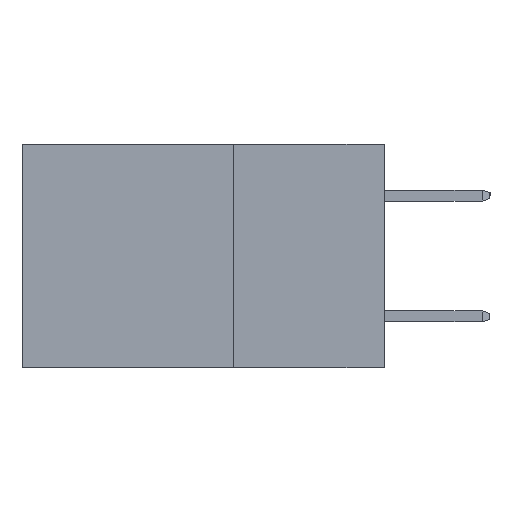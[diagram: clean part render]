
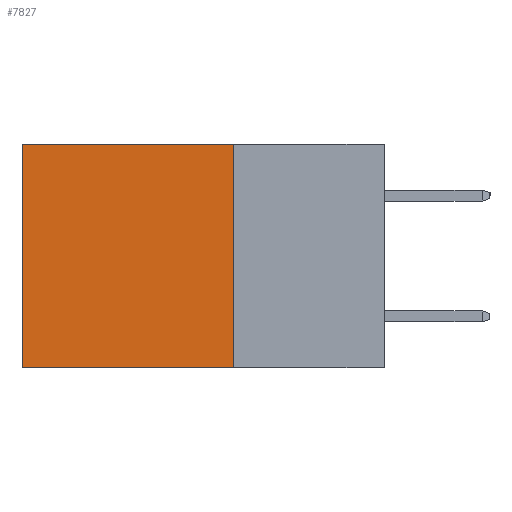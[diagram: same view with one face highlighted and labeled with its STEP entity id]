
A CAD part, left-side view. The second image highlights one B-rep face of the part: STEP entity #7827.
In plain terms, the highlighted planar face has unit normal (-1, 0, 0).
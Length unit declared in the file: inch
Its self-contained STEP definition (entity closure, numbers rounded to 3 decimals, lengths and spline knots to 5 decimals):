
#541 = VECTOR ( 'NONE', #6276, 39.37008 ) ;
#549 = CARTESIAN_POINT ( 'NONE',  ( 0.2615, 0.25, -0.37 ) ) ;
#637 = VERTEX_POINT ( 'NONE', #14362 ) ;
#1221 = VERTEX_POINT ( 'NONE', #3086 ) ;
#1409 = LINE ( 'NONE', #11494, #1584 ) ;
#1584 = VECTOR ( 'NONE', #2761, 39.37008 ) ;
#1722 = AXIS2_PLACEMENT_3D ( 'NONE', #14003, #3047, #11339 ) ;
#1917 = CARTESIAN_POINT ( 'NONE',  ( 0.2615, 0.6, 0. ) ) ;
#2754 = ORIENTED_EDGE ( 'NONE', *, *, #12597, .F. ) ;
#2761 = DIRECTION ( 'NONE',  ( 0., 0., -1. ) ) ;
#3027 = EDGE_LOOP ( 'NONE', ( #10962, #6951, #2754, #10366 ) ) ;
#3047 = DIRECTION ( 'NONE',  ( 1., 0., 0. ) ) ;
#3086 = CARTESIAN_POINT ( 'NONE',  ( 0.2615, 0.25, 0. ) ) ;
#3855 = VECTOR ( 'NONE', #7475, 39.37008 ) ;
#4881 = FACE_OUTER_BOUND ( 'NONE', #3027, .T. ) ;
#5173 = EDGE_CURVE ( 'NONE', #9083, #7657, #5642, .T. ) ;
#5642 = LINE ( 'NONE', #9201, #6374 ) ;
#6276 = DIRECTION ( 'NONE',  ( 0., 1., 0. ) ) ;
#6352 = LINE ( 'NONE', #549, #541 ) ;
#6374 = VECTOR ( 'NONE', #9130, 39.37008 ) ;
#6568 = EDGE_CURVE ( 'NONE', #1221, #9083, #11397, .T. ) ;
#6951 = ORIENTED_EDGE ( 'NONE', *, *, #13438, .F. ) ;
#7475 = DIRECTION ( 'NONE',  ( 0., 1., 0. ) ) ;
#7657 = VERTEX_POINT ( 'NONE', #10856 ) ;
#7827 = ADVANCED_FACE ( 'NONE', ( #4881 ), #9564, .F. ) ;
#9083 = VERTEX_POINT ( 'NONE', #1917 ) ;
#9130 = DIRECTION ( 'NONE',  ( 0., 0., -1. ) ) ;
#9201 = CARTESIAN_POINT ( 'NONE',  ( 0.2615, 0.6, -0.37 ) ) ;
#9564 = PLANE ( 'NONE',  #1722 ) ;
#10366 = ORIENTED_EDGE ( 'NONE', *, *, #6568, .T. ) ;
#10856 = CARTESIAN_POINT ( 'NONE',  ( 0.2615, 0.6, -0.37 ) ) ;
#10962 = ORIENTED_EDGE ( 'NONE', *, *, #5173, .T. ) ;
#11339 = DIRECTION ( 'NONE',  ( 0., 0., -1. ) ) ;
#11397 = LINE ( 'NONE', #12442, #3855 ) ;
#11494 = CARTESIAN_POINT ( 'NONE',  ( 0.2615, 0.25, -0.37 ) ) ;
#12442 = CARTESIAN_POINT ( 'NONE',  ( 0.2615, 0.25, 0. ) ) ;
#12597 = EDGE_CURVE ( 'NONE', #1221, #637, #1409, .T. ) ;
#13438 = EDGE_CURVE ( 'NONE', #637, #7657, #6352, .T. ) ;
#14003 = CARTESIAN_POINT ( 'NONE',  ( 0.2615, 0.25, -0.37 ) ) ;
#14362 = CARTESIAN_POINT ( 'NONE',  ( 0.2615, 0.25, -0.37 ) ) ;
